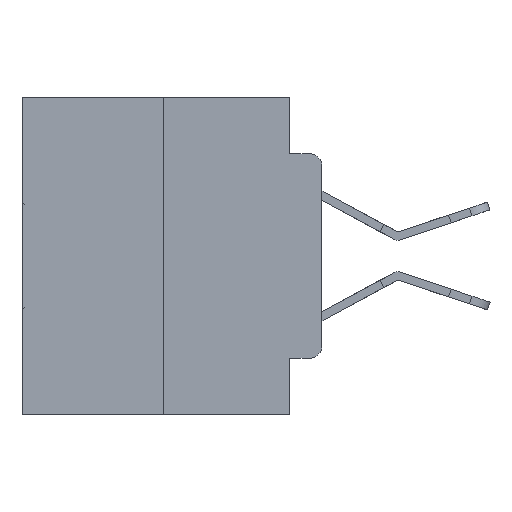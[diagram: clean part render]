
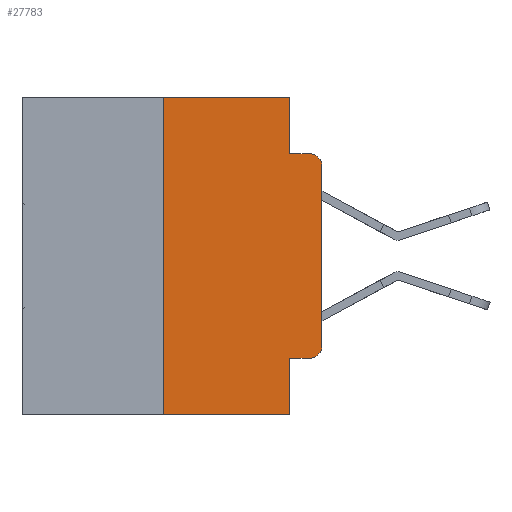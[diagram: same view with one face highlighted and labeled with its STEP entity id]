
A CAD part, left-side view. The second image highlights one B-rep face of the part: STEP entity #27783.
In plain terms, the highlighted planar face has unit normal (-1, 0, 0).
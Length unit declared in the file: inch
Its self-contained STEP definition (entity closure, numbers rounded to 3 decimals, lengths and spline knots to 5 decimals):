
#430 = CARTESIAN_POINT ( 'NONE',  ( 0., 0.02, -0.4115 ) ) ;
#790 = AXIS2_PLACEMENT_3D ( 'NONE', #29503, #26993, #29608 ) ;
#1039 = LINE ( 'NONE', #19227, #25115 ) ;
#1058 = EDGE_CURVE ( 'NONE', #25237, #23398, #1176, .T. ) ;
#1176 = LINE ( 'NONE', #31645, #22130 ) ;
#1563 = ORIENTED_EDGE ( 'NONE', *, *, #1058, .F. ) ;
#1630 = DIRECTION ( 'NONE',  ( 0., 0., 1. ) ) ;
#2203 = EDGE_CURVE ( 'NONE', #8816, #18194, #25550, .T. ) ;
#3118 = LINE ( 'NONE', #5912, #31490 ) ;
#4092 = CARTESIAN_POINT ( 'NONE',  ( 0., 0.02, -0.3915 ) ) ;
#5027 = CIRCLE ( 'NONE', #790, 0.02 ) ;
#5151 = VERTEX_POINT ( 'NONE', #29109 ) ;
#5731 = DIRECTION ( 'NONE',  ( 1., 0., 0. ) ) ;
#5912 = CARTESIAN_POINT ( 'NONE',  ( 0., 0.473, -0.5 ) ) ;
#6261 = ORIENTED_EDGE ( 'NONE', *, *, #14973, .F. ) ;
#6991 = CARTESIAN_POINT ( 'NONE',  ( 0., 0.051, 0. ) ) ;
#7448 = CARTESIAN_POINT ( 'NONE',  ( 0., 0.051, 0. ) ) ;
#7817 = ORIENTED_EDGE ( 'NONE', *, *, #12001, .F. ) ;
#8327 = VECTOR ( 'NONE', #31357, 39.37008 ) ;
#8549 = CARTESIAN_POINT ( 'NONE',  ( 0., 0.473, 0. ) ) ;
#8816 = VERTEX_POINT ( 'NONE', #26476 ) ;
#9225 = LINE ( 'NONE', #7448, #23200 ) ;
#9333 = EDGE_CURVE ( 'NONE', #27436, #31245, #3118, .T. ) ;
#11045 = VECTOR ( 'NONE', #13724, 39.37008 ) ;
#11230 = VECTOR ( 'NONE', #11371, 39.37008 ) ;
#11371 = DIRECTION ( 'NONE',  ( 0., -1., 0. ) ) ;
#11725 = DIRECTION ( 'NONE',  ( -1., 0., 0. ) ) ;
#12001 = EDGE_CURVE ( 'NONE', #17913, #5151, #14822, .T. ) ;
#12571 = VERTEX_POINT ( 'NONE', #31287 ) ;
#13344 = EDGE_CURVE ( 'NONE', #22003, #23398, #5027, .T. ) ;
#13724 = DIRECTION ( 'NONE',  ( 0., 0., 1. ) ) ;
#14474 = CARTESIAN_POINT ( 'NONE',  ( 0., 0.25, 0. ) ) ;
#14822 = LINE ( 'NONE', #29299, #22136 ) ;
#14973 = EDGE_CURVE ( 'NONE', #27436, #17913, #1039, .T. ) ;
#16175 = EDGE_CURVE ( 'NONE', #5151, #25237, #31297, .T. ) ;
#16310 = ORIENTED_EDGE ( 'NONE', *, *, #16605, .T. ) ;
#16605 = EDGE_CURVE ( 'NONE', #12571, #22003, #23424, .T. ) ;
#16872 = CARTESIAN_POINT ( 'NONE',  ( 0., 0.25, -0.5 ) ) ;
#16874 = CIRCLE ( 'NONE', #28213, 0.02 ) ;
#17913 = VERTEX_POINT ( 'NONE', #14474 ) ;
#18194 = VERTEX_POINT ( 'NONE', #430 ) ;
#18839 = DIRECTION ( 'NONE',  ( 0., -1., 0. ) ) ;
#19227 = CARTESIAN_POINT ( 'NONE',  ( 0., 0.25, 0. ) ) ;
#19574 = ORIENTED_EDGE ( 'NONE', *, *, #30522, .T. ) ;
#20519 = FACE_OUTER_BOUND ( 'NONE', #22102, .T. ) ;
#20593 = DIRECTION ( 'NONE',  ( 0., 0., -1. ) ) ;
#22003 = VERTEX_POINT ( 'NONE', #28800 ) ;
#22102 = EDGE_LOOP ( 'NONE', ( #16310, #27624, #1563, #22856, #7817, #6261, #28291, #29111, #30278, #19574 ) ) ;
#22130 = VECTOR ( 'NONE', #18839, 39.37008 ) ;
#22136 = VECTOR ( 'NONE', #31691, 39.37008 ) ;
#22509 = CARTESIAN_POINT ( 'NONE',  ( 0., 0.051, -0.5 ) ) ;
#22856 = ORIENTED_EDGE ( 'NONE', *, *, #16175, .F. ) ;
#23160 = AXIS2_PLACEMENT_3D ( 'NONE', #8549, #5731, #23197 ) ;
#23197 = DIRECTION ( 'NONE',  ( 0., 0., -1. ) ) ;
#23200 = VECTOR ( 'NONE', #20593, 39.37008 ) ;
#23398 = VERTEX_POINT ( 'NONE', #27562 ) ;
#23424 = LINE ( 'NONE', #28573, #11045 ) ;
#25115 = VECTOR ( 'NONE', #1630, 39.37008 ) ;
#25237 = VERTEX_POINT ( 'NONE', #26677 ) ;
#25550 = LINE ( 'NONE', #28077, #11230 ) ;
#26476 = CARTESIAN_POINT ( 'NONE',  ( 0., 0.051, -0.4115 ) ) ;
#26677 = CARTESIAN_POINT ( 'NONE',  ( 0., 0.051, -0.0885 ) ) ;
#26993 = DIRECTION ( 'NONE',  ( -1., 0., 0. ) ) ;
#27046 = DIRECTION ( 'NONE',  ( 0., -1., 0. ) ) ;
#27436 = VERTEX_POINT ( 'NONE', #16872 ) ;
#27562 = CARTESIAN_POINT ( 'NONE',  ( 0., 0.02, -0.0885 ) ) ;
#27624 = ORIENTED_EDGE ( 'NONE', *, *, #13344, .T. ) ;
#27783 = ADVANCED_FACE ( 'NONE', ( #20519 ), #30517, .F. ) ;
#28077 = CARTESIAN_POINT ( 'NONE',  ( 0., 0.051, -0.4115 ) ) ;
#28164 = EDGE_CURVE ( 'NONE', #8816, #31245, #9225, .T. ) ;
#28213 = AXIS2_PLACEMENT_3D ( 'NONE', #4092, #11725, #31608 ) ;
#28291 = ORIENTED_EDGE ( 'NONE', *, *, #9333, .T. ) ;
#28573 = CARTESIAN_POINT ( 'NONE',  ( 0., 0., 0. ) ) ;
#28800 = CARTESIAN_POINT ( 'NONE',  ( 0., 0., -0.1085 ) ) ;
#29109 = CARTESIAN_POINT ( 'NONE',  ( 0., 0.051, 0. ) ) ;
#29111 = ORIENTED_EDGE ( 'NONE', *, *, #28164, .F. ) ;
#29299 = CARTESIAN_POINT ( 'NONE',  ( 0., 0.473, 0. ) ) ;
#29503 = CARTESIAN_POINT ( 'NONE',  ( 0., 0.02, -0.1085 ) ) ;
#29608 = DIRECTION ( 'NONE',  ( 0., 0., -1. ) ) ;
#30278 = ORIENTED_EDGE ( 'NONE', *, *, #2203, .T. ) ;
#30517 = PLANE ( 'NONE',  #23160 ) ;
#30522 = EDGE_CURVE ( 'NONE', #18194, #12571, #16874, .T. ) ;
#31245 = VERTEX_POINT ( 'NONE', #22509 ) ;
#31287 = CARTESIAN_POINT ( 'NONE',  ( 0., 0., -0.3915 ) ) ;
#31297 = LINE ( 'NONE', #6991, #8327 ) ;
#31357 = DIRECTION ( 'NONE',  ( 0., 0., -1. ) ) ;
#31490 = VECTOR ( 'NONE', #27046, 39.37008 ) ;
#31608 = DIRECTION ( 'NONE',  ( 0., 0., -1. ) ) ;
#31645 = CARTESIAN_POINT ( 'NONE',  ( 0., 0.051, -0.0885 ) ) ;
#31691 = DIRECTION ( 'NONE',  ( 0., -1., 0. ) ) ;
